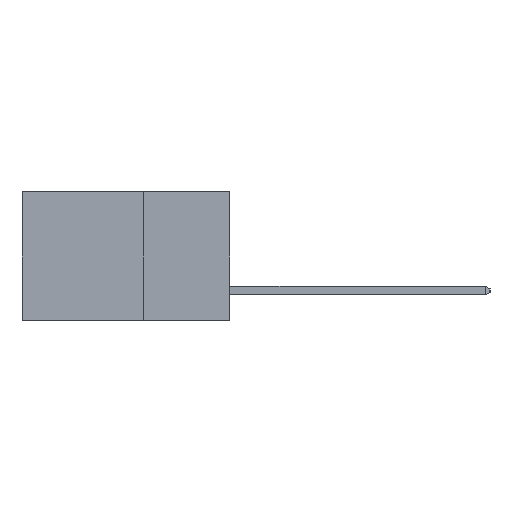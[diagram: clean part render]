
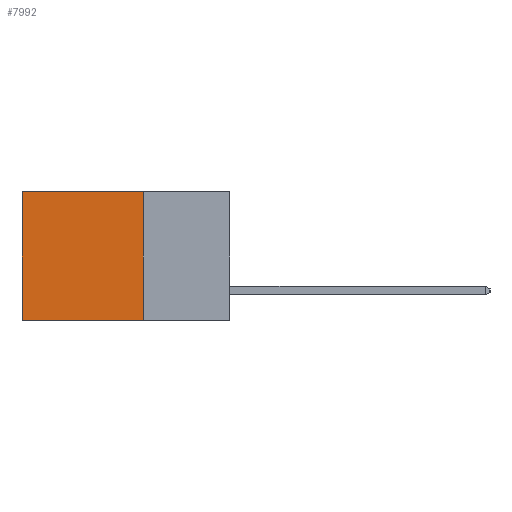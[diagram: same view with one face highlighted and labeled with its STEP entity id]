
A CAD part, left-side view. The second image highlights one B-rep face of the part: STEP entity #7992.
In plain terms, the highlighted planar face has unit normal (-1, 0, 0).
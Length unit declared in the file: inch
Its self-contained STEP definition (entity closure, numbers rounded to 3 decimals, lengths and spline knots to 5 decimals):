
#185 = DIRECTION ( 'NONE',  ( 0., 1., 0. ) ) ;
#497 = DIRECTION ( 'NONE',  ( 0., 1., 0. ) ) ;
#3519 = EDGE_CURVE ( 'NONE', #14670, #5757, #12906, .T. ) ;
#3530 = CARTESIAN_POINT ( 'NONE',  ( 0.2615, 0.6, -0.37 ) ) ;
#3684 = VECTOR ( 'NONE', #8741, 39.37008 ) ;
#3795 = AXIS2_PLACEMENT_3D ( 'NONE', #5703, #4503, #12907 ) ;
#4126 = LINE ( 'NONE', #14715, #13704 ) ;
#4495 = CARTESIAN_POINT ( 'NONE',  ( 0.2615, 0.25, -0.37 ) ) ;
#4503 = DIRECTION ( 'NONE',  ( 1., 0., 0. ) ) ;
#4548 = CARTESIAN_POINT ( 'NONE',  ( 0.2615, 0.6, 0. ) ) ;
#4623 = ORIENTED_EDGE ( 'NONE', *, *, #3519, .T. ) ;
#5145 = VECTOR ( 'NONE', #6908, 39.37008 ) ;
#5244 = FACE_OUTER_BOUND ( 'NONE', #5820, .T. ) ;
#5703 = CARTESIAN_POINT ( 'NONE',  ( 0.2615, 0.25, -0.37 ) ) ;
#5757 = VERTEX_POINT ( 'NONE', #3530 ) ;
#5820 = EDGE_LOOP ( 'NONE', ( #4623, #7008, #7258, #6396 ) ) ;
#6184 = VERTEX_POINT ( 'NONE', #6748 ) ;
#6396 = ORIENTED_EDGE ( 'NONE', *, *, #7184, .T. ) ;
#6748 = CARTESIAN_POINT ( 'NONE',  ( 0.2615, 0.25, 0. ) ) ;
#6908 = DIRECTION ( 'NONE',  ( 0., 0., -1. ) ) ;
#7008 = ORIENTED_EDGE ( 'NONE', *, *, #7325, .F. ) ;
#7184 = EDGE_CURVE ( 'NONE', #6184, #14670, #4126, .T. ) ;
#7258 = ORIENTED_EDGE ( 'NONE', *, *, #14616, .F. ) ;
#7325 = EDGE_CURVE ( 'NONE', #11886, #5757, #11481, .T. ) ;
#7992 = ADVANCED_FACE ( 'NONE', ( #5244 ), #8066, .F. ) ;
#8066 = PLANE ( 'NONE',  #3795 ) ;
#8302 = VECTOR ( 'NONE', #497, 39.37008 ) ;
#8377 = LINE ( 'NONE', #4495, #5145 ) ;
#8741 = DIRECTION ( 'NONE',  ( 0., 0., -1. ) ) ;
#8791 = CARTESIAN_POINT ( 'NONE',  ( 0.2615, 0.6, -0.37 ) ) ;
#11481 = LINE ( 'NONE', #13795, #8302 ) ;
#11886 = VERTEX_POINT ( 'NONE', #13773 ) ;
#12906 = LINE ( 'NONE', #8791, #3684 ) ;
#12907 = DIRECTION ( 'NONE',  ( 0., 0., -1. ) ) ;
#13704 = VECTOR ( 'NONE', #185, 39.37008 ) ;
#13773 = CARTESIAN_POINT ( 'NONE',  ( 0.2615, 0.25, -0.37 ) ) ;
#13795 = CARTESIAN_POINT ( 'NONE',  ( 0.2615, 0.25, -0.37 ) ) ;
#14616 = EDGE_CURVE ( 'NONE', #6184, #11886, #8377, .T. ) ;
#14670 = VERTEX_POINT ( 'NONE', #4548 ) ;
#14715 = CARTESIAN_POINT ( 'NONE',  ( 0.2615, 0.25, 0. ) ) ;
